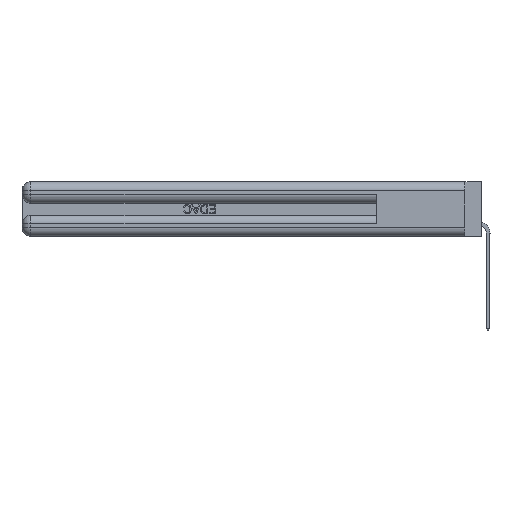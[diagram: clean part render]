
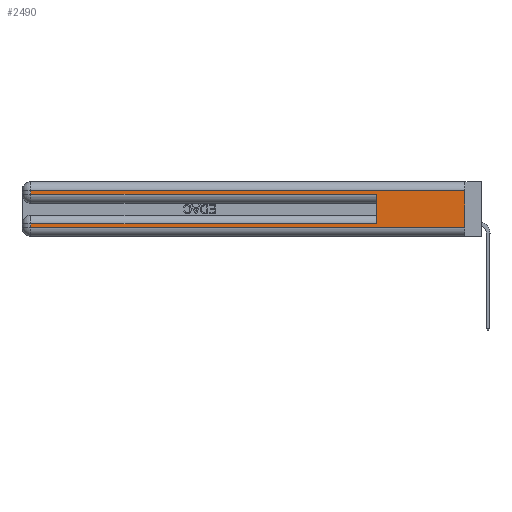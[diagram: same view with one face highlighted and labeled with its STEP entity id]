
A CAD part, left-side view. The second image highlights one B-rep face of the part: STEP entity #2490.
In plain terms, the highlighted planar face has unit normal (-1, 0, 0).
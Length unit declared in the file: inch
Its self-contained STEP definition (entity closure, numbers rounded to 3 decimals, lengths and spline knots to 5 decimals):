
#235 = LINE ( 'NONE', #18718, #42035 ) ;
#970 = ORIENTED_EDGE ( 'NONE', *, *, #15952, .T. ) ;
#1629 = VERTEX_POINT ( 'NONE', #34439 ) ;
#2490 = ADVANCED_FACE ( 'NONE', ( #39542 ), #28503, .F. ) ;
#5345 = DIRECTION ( 'NONE',  ( 0., 0., -1. ) ) ;
#5886 = DIRECTION ( 'NONE',  ( 0., -1., 0. ) ) ;
#5889 = CARTESIAN_POINT ( 'NONE',  ( 0., 2.94, 0.31 ) ) ;
#5937 = ORIENTED_EDGE ( 'NONE', *, *, #34521, .F. ) ;
#7817 = LINE ( 'NONE', #8349, #29093 ) ;
#8349 = CARTESIAN_POINT ( 'NONE',  ( 0., 2.94, 0.37 ) ) ;
#9435 = ORIENTED_EDGE ( 'NONE', *, *, #17772, .T. ) ;
#11223 = ORIENTED_EDGE ( 'NONE', *, *, #40661, .F. ) ;
#12496 = VECTOR ( 'NONE', #23079, 39.37008 ) ;
#12525 = CARTESIAN_POINT ( 'NONE',  ( 0., 0.6, 0.285 ) ) ;
#13251 = CARTESIAN_POINT ( 'NONE',  ( 0., 2.94, 0.06 ) ) ;
#13925 = VECTOR ( 'NONE', #19517, 39.37008 ) ;
#15088 = EDGE_CURVE ( 'NONE', #18270, #41087, #7817, .T. ) ;
#15165 = EDGE_LOOP ( 'NONE', ( #5937, #36671, #24244, #970, #11223, #16419, #9435, #25333 ) ) ;
#15952 = EDGE_CURVE ( 'NONE', #41087, #27415, #23852, .T. ) ;
#16419 = ORIENTED_EDGE ( 'NONE', *, *, #42200, .T. ) ;
#17772 = EDGE_CURVE ( 'NONE', #43147, #39097, #235, .T. ) ;
#18270 = VERTEX_POINT ( 'NONE', #5889 ) ;
#18424 = DIRECTION ( 'NONE',  ( 1., 0., 0. ) ) ;
#18718 = CARTESIAN_POINT ( 'NONE',  ( 0., 2.94, 0.37 ) ) ;
#18828 = CARTESIAN_POINT ( 'NONE',  ( 0., 0., 0.37 ) ) ;
#19076 = AXIS2_PLACEMENT_3D ( 'NONE', #18828, #18424, #5345 ) ;
#19517 = DIRECTION ( 'NONE',  ( 0., 0., 1. ) ) ;
#19563 = LINE ( 'NONE', #29404, #42063 ) ;
#22301 = CARTESIAN_POINT ( 'NONE',  ( 0., 0., 0.31 ) ) ;
#22845 = CARTESIAN_POINT ( 'NONE',  ( 0., 0., 0.06 ) ) ;
#23079 = DIRECTION ( 'NONE',  ( 0., 0., -1. ) ) ;
#23595 = VERTEX_POINT ( 'NONE', #22845 ) ;
#23852 = LINE ( 'NONE', #42503, #33690 ) ;
#24244 = ORIENTED_EDGE ( 'NONE', *, *, #15088, .T. ) ;
#25333 = ORIENTED_EDGE ( 'NONE', *, *, #40631, .T. ) ;
#25534 = DIRECTION ( 'NONE',  ( 0., -1., 0. ) ) ;
#25887 = CARTESIAN_POINT ( 'NONE',  ( 0., 2.94, 0.285 ) ) ;
#26387 = DIRECTION ( 'NONE',  ( 0., 1., 0. ) ) ;
#26408 = CARTESIAN_POINT ( 'NONE',  ( 0., 0., 0.37 ) ) ;
#27287 = CARTESIAN_POINT ( 'NONE',  ( 0., 2.94, 0.085 ) ) ;
#27312 = LINE ( 'NONE', #30530, #42053 ) ;
#27415 = VERTEX_POINT ( 'NONE', #12525 ) ;
#28503 = PLANE ( 'NONE',  #19076 ) ;
#28895 = VERTEX_POINT ( 'NONE', #22301 ) ;
#29093 = VECTOR ( 'NONE', #34343, 39.37008 ) ;
#29383 = EDGE_CURVE ( 'NONE', #28895, #18270, #27312, .T. ) ;
#29404 = CARTESIAN_POINT ( 'NONE',  ( 0., 0., 0.085 ) ) ;
#29490 = VECTOR ( 'NONE', #5886, 39.37008 ) ;
#30530 = CARTESIAN_POINT ( 'NONE',  ( 0., 0., 0.31 ) ) ;
#32982 = CARTESIAN_POINT ( 'NONE',  ( 0., 0.6, 0.145 ) ) ;
#33690 = VECTOR ( 'NONE', #25534, 39.37008 ) ;
#34343 = DIRECTION ( 'NONE',  ( 0., 0., -1. ) ) ;
#34344 = DIRECTION ( 'NONE',  ( 0., 1., 0. ) ) ;
#34439 = CARTESIAN_POINT ( 'NONE',  ( 0., 0.6, 0.085 ) ) ;
#34521 = EDGE_CURVE ( 'NONE', #28895, #23595, #43206, .T. ) ;
#35101 = DIRECTION ( 'NONE',  ( 0., 0., -1. ) ) ;
#35378 = CARTESIAN_POINT ( 'NONE',  ( 0., 0., 0.06 ) ) ;
#36671 = ORIENTED_EDGE ( 'NONE', *, *, #29383, .T. ) ;
#39097 = VERTEX_POINT ( 'NONE', #13251 ) ;
#39542 = FACE_OUTER_BOUND ( 'NONE', #15165, .T. ) ;
#40570 = LINE ( 'NONE', #35378, #29490 ) ;
#40631 = EDGE_CURVE ( 'NONE', #39097, #23595, #40570, .T. ) ;
#40661 = EDGE_CURVE ( 'NONE', #1629, #27415, #42662, .T. ) ;
#41087 = VERTEX_POINT ( 'NONE', #25887 ) ;
#42035 = VECTOR ( 'NONE', #35101, 39.37008 ) ;
#42053 = VECTOR ( 'NONE', #34344, 39.37008 ) ;
#42063 = VECTOR ( 'NONE', #26387, 39.37008 ) ;
#42200 = EDGE_CURVE ( 'NONE', #1629, #43147, #19563, .T. ) ;
#42503 = CARTESIAN_POINT ( 'NONE',  ( 0., 0., 0.285 ) ) ;
#42662 = LINE ( 'NONE', #32982, #13925 ) ;
#43147 = VERTEX_POINT ( 'NONE', #27287 ) ;
#43206 = LINE ( 'NONE', #26408, #12496 ) ;
